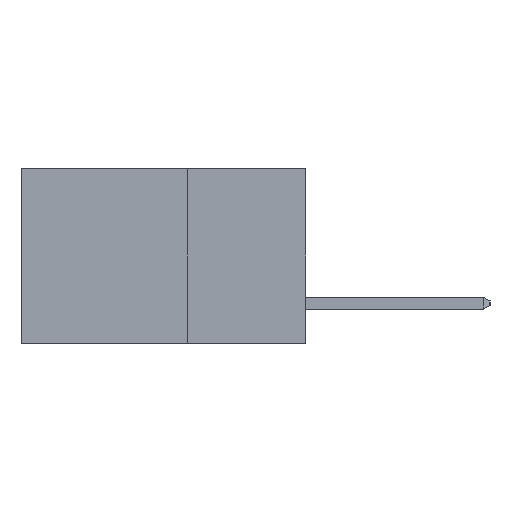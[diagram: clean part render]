
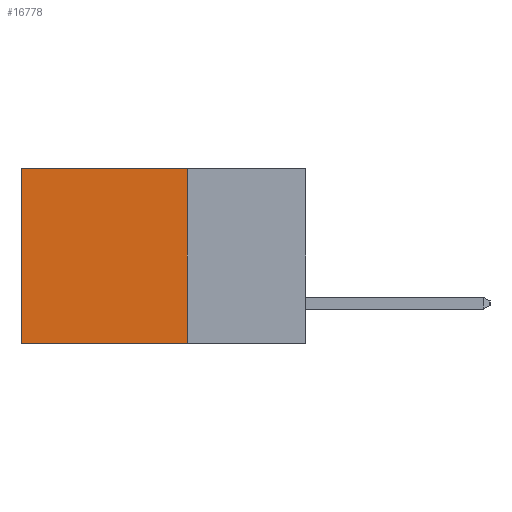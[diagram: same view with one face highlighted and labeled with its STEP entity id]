
A CAD part, left-side view. The second image highlights one B-rep face of the part: STEP entity #16778.
In plain terms, the highlighted planar face has unit normal (-1, 0, 0).
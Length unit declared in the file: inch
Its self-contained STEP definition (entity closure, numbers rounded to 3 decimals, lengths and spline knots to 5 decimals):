
#448 = CARTESIAN_POINT ( 'NONE',  ( 0.298, 0.25, 0. ) ) ;
#1458 = VECTOR ( 'NONE', #2795, 39.37008 ) ;
#1602 = VECTOR ( 'NONE', #2556, 39.37008 ) ;
#2556 = DIRECTION ( 'NONE',  ( 0., 1., 0. ) ) ;
#2599 = EDGE_CURVE ( 'NONE', #7765, #8090, #19219, .T. ) ;
#2795 = DIRECTION ( 'NONE',  ( 0., 0., -1. ) ) ;
#4456 = ORIENTED_EDGE ( 'NONE', *, *, #11500, .T. ) ;
#5045 = VECTOR ( 'NONE', #6126, 39.37008 ) ;
#5211 = CARTESIAN_POINT ( 'NONE',  ( 0.298, 0.25, -0.37 ) ) ;
#5505 = DIRECTION ( 'NONE',  ( 1., 0., 0. ) ) ;
#6063 = ORIENTED_EDGE ( 'NONE', *, *, #2599, .F. ) ;
#6126 = DIRECTION ( 'NONE',  ( 0., 1., 0. ) ) ;
#6161 = VECTOR ( 'NONE', #16555, 39.37008 ) ;
#6533 = EDGE_CURVE ( 'NONE', #13198, #7765, #19076, .T. ) ;
#7765 = VERTEX_POINT ( 'NONE', #15938 ) ;
#7860 = CARTESIAN_POINT ( 'NONE',  ( 0.298, 0.25, 0. ) ) ;
#8090 = VERTEX_POINT ( 'NONE', #17227 ) ;
#8536 = ORIENTED_EDGE ( 'NONE', *, *, #8780, .T. ) ;
#8574 = AXIS2_PLACEMENT_3D ( 'NONE', #13724, #5505, #17149 ) ;
#8780 = EDGE_CURVE ( 'NONE', #13198, #12275, #17251, .T. ) ;
#10530 = CARTESIAN_POINT ( 'NONE',  ( 0.298, 0.25, 0. ) ) ;
#11500 = EDGE_CURVE ( 'NONE', #12275, #8090, #19394, .T. ) ;
#11507 = CARTESIAN_POINT ( 'NONE',  ( 0.298, 0.6, 0. ) ) ;
#12275 = VERTEX_POINT ( 'NONE', #11507 ) ;
#13063 = FACE_OUTER_BOUND ( 'NONE', #20960, .T. ) ;
#13198 = VERTEX_POINT ( 'NONE', #448 ) ;
#13724 = CARTESIAN_POINT ( 'NONE',  ( 0.298, 0.25, 0. ) ) ;
#14941 = CARTESIAN_POINT ( 'NONE',  ( 0.298, 0.6, 0. ) ) ;
#15527 = PLANE ( 'NONE',  #8574 ) ;
#15653 = ORIENTED_EDGE ( 'NONE', *, *, #6533, .F. ) ;
#15938 = CARTESIAN_POINT ( 'NONE',  ( 0.298, 0.25, -0.37 ) ) ;
#16555 = DIRECTION ( 'NONE',  ( 0., 0., -1. ) ) ;
#16778 = ADVANCED_FACE ( 'NONE', ( #13063 ), #15527, .F. ) ;
#17149 = DIRECTION ( 'NONE',  ( 0., 0., -1. ) ) ;
#17227 = CARTESIAN_POINT ( 'NONE',  ( 0.298, 0.6, -0.37 ) ) ;
#17251 = LINE ( 'NONE', #7860, #5045 ) ;
#19076 = LINE ( 'NONE', #10530, #1458 ) ;
#19219 = LINE ( 'NONE', #5211, #1602 ) ;
#19394 = LINE ( 'NONE', #14941, #6161 ) ;
#20960 = EDGE_LOOP ( 'NONE', ( #4456, #6063, #15653, #8536 ) ) ;
